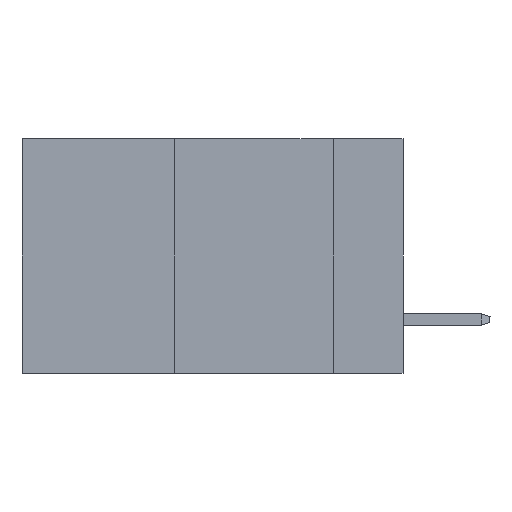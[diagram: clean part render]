
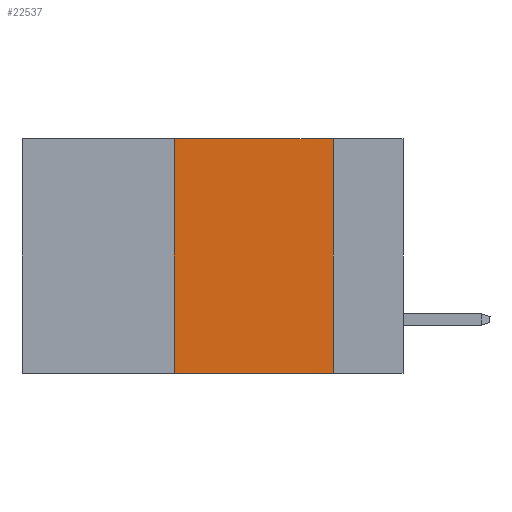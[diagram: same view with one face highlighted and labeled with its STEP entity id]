
A CAD part, left-side view. The second image highlights one B-rep face of the part: STEP entity #22537.
In plain terms, the highlighted planar face has unit normal (-1, 0, 0).
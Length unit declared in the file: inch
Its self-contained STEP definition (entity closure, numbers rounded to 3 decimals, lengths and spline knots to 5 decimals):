
#497 = ORIENTED_EDGE ( 'NONE', *, *, #16158, .F. ) ;
#509 = VECTOR ( 'NONE', #15194, 39.37008 ) ;
#667 = EDGE_CURVE ( 'NONE', #19381, #4712, #10547, .T. ) ;
#1007 = EDGE_CURVE ( 'NONE', #4712, #2959, #5045, .T. ) ;
#1653 = ORIENTED_EDGE ( 'NONE', *, *, #1007, .F. ) ;
#1855 = PLANE ( 'NONE',  #4921 ) ;
#2355 = LINE ( 'NONE', #9455, #509 ) ;
#2959 = VERTEX_POINT ( 'NONE', #12738 ) ;
#2977 = CARTESIAN_POINT ( 'NONE',  ( 0., 0.11, -0.37 ) ) ;
#3318 = DIRECTION ( 'NONE',  ( 0., 0., 1. ) ) ;
#3322 = CARTESIAN_POINT ( 'NONE',  ( 0., 0.11, 0. ) ) ;
#4712 = VERTEX_POINT ( 'NONE', #6455 ) ;
#4921 = AXIS2_PLACEMENT_3D ( 'NONE', #18217, #7576, #16240 ) ;
#4933 = DIRECTION ( 'NONE',  ( 0., -1., 0. ) ) ;
#5045 = LINE ( 'NONE', #14055, #16592 ) ;
#6019 = VECTOR ( 'NONE', #8805, 39.37008 ) ;
#6455 = CARTESIAN_POINT ( 'NONE',  ( 0., 0.36, 0. ) ) ;
#6693 = CARTESIAN_POINT ( 'NONE',  ( 0., 0.36, 0. ) ) ;
#7576 = DIRECTION ( 'NONE',  ( 1., 0., 0. ) ) ;
#8553 = ORIENTED_EDGE ( 'NONE', *, *, #667, .F. ) ;
#8805 = DIRECTION ( 'NONE',  ( 0., 0., -1. ) ) ;
#9455 = CARTESIAN_POINT ( 'NONE',  ( 0., 0.6, -0.37 ) ) ;
#10547 = LINE ( 'NONE', #6693, #17706 ) ;
#11436 = CARTESIAN_POINT ( 'NONE',  ( 0., 0.36, -0.37 ) ) ;
#12738 = CARTESIAN_POINT ( 'NONE',  ( 0., 0.11, 0. ) ) ;
#14055 = CARTESIAN_POINT ( 'NONE',  ( 0., 0.6, 0. ) ) ;
#14314 = EDGE_LOOP ( 'NONE', ( #497, #1653, #8553, #22323 ) ) ;
#15194 = DIRECTION ( 'NONE',  ( 0., -1., 0. ) ) ;
#16158 = EDGE_CURVE ( 'NONE', #2959, #17121, #17704, .T. ) ;
#16240 = DIRECTION ( 'NONE',  ( 0., 0., -1. ) ) ;
#16592 = VECTOR ( 'NONE', #4933, 39.37008 ) ;
#17121 = VERTEX_POINT ( 'NONE', #2977 ) ;
#17704 = LINE ( 'NONE', #3322, #6019 ) ;
#17706 = VECTOR ( 'NONE', #3318, 39.37008 ) ;
#18000 = FACE_OUTER_BOUND ( 'NONE', #14314, .T. ) ;
#18073 = EDGE_CURVE ( 'NONE', #19381, #17121, #2355, .T. ) ;
#18217 = CARTESIAN_POINT ( 'NONE',  ( 0., 0.6, 0. ) ) ;
#19381 = VERTEX_POINT ( 'NONE', #11436 ) ;
#22323 = ORIENTED_EDGE ( 'NONE', *, *, #18073, .T. ) ;
#22537 = ADVANCED_FACE ( 'NONE', ( #18000 ), #1855, .F. ) ;
